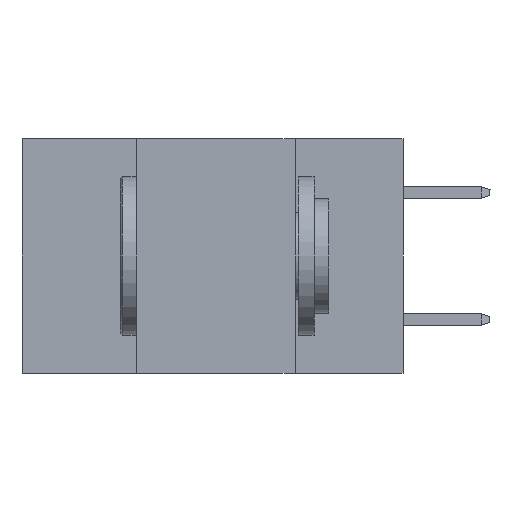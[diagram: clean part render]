
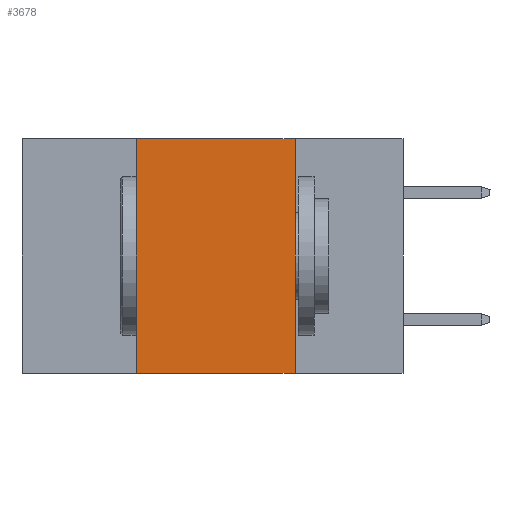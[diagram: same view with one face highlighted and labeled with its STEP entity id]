
A CAD part, left-side view. The second image highlights one B-rep face of the part: STEP entity #3678.
In plain terms, the highlighted planar face has unit normal (-1, 0, 0).
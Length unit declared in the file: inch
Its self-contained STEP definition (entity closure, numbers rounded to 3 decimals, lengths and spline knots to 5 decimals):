
#543 = ORIENTED_EDGE ( 'NONE', *, *, #1436, .F. ) ;
#1436 = EDGE_CURVE ( 'NONE', #8784, #13768, #17062, .T. ) ;
#1684 = DIRECTION ( 'NONE',  ( 1., 0., 0. ) ) ;
#2003 = CARTESIAN_POINT ( 'NONE',  ( 0., 0.42, 0. ) ) ;
#2241 = CARTESIAN_POINT ( 'NONE',  ( 0., 0.6, 0. ) ) ;
#2325 = EDGE_CURVE ( 'NONE', #8310, #11814, #17284, .T. ) ;
#3015 = PLANE ( 'NONE',  #15207 ) ;
#3678 = ADVANCED_FACE ( 'NONE', ( #11215 ), #3015, .F. ) ;
#4922 = LINE ( 'NONE', #2241, #7880 ) ;
#5837 = CARTESIAN_POINT ( 'NONE',  ( 0., 0.6, -0.37 ) ) ;
#6354 = VECTOR ( 'NONE', #16234, 39.37008 ) ;
#6727 = ORIENTED_EDGE ( 'NONE', *, *, #2325, .F. ) ;
#6838 = VECTOR ( 'NONE', #12905, 39.37008 ) ;
#7275 = ORIENTED_EDGE ( 'NONE', *, *, #7695, .T. ) ;
#7695 = EDGE_CURVE ( 'NONE', #8784, #11814, #16608, .T. ) ;
#7716 = DIRECTION ( 'NONE',  ( 0., -1., 0. ) ) ;
#7880 = VECTOR ( 'NONE', #7716, 39.37008 ) ;
#8310 = VERTEX_POINT ( 'NONE', #11149 ) ;
#8784 = VERTEX_POINT ( 'NONE', #8899 ) ;
#8899 = CARTESIAN_POINT ( 'NONE',  ( 0., 0.42, -0.37 ) ) ;
#9472 = CARTESIAN_POINT ( 'NONE',  ( 0., 0.17, 0. ) ) ;
#9924 = DIRECTION ( 'NONE',  ( 0., -1., 0. ) ) ;
#9996 = CARTESIAN_POINT ( 'NONE',  ( 0., 0.17, -0.37 ) ) ;
#10149 = CARTESIAN_POINT ( 'NONE',  ( 0., 0.6, 0. ) ) ;
#10281 = ORIENTED_EDGE ( 'NONE', *, *, #10549, .F. ) ;
#10549 = EDGE_CURVE ( 'NONE', #13768, #8310, #4922, .T. ) ;
#11149 = CARTESIAN_POINT ( 'NONE',  ( 0., 0.17, 0. ) ) ;
#11215 = FACE_OUTER_BOUND ( 'NONE', #13822, .T. ) ;
#11299 = DIRECTION ( 'NONE',  ( 0., 0., -1. ) ) ;
#11814 = VERTEX_POINT ( 'NONE', #9996 ) ;
#12905 = DIRECTION ( 'NONE',  ( 0., 0., 1. ) ) ;
#13768 = VERTEX_POINT ( 'NONE', #15091 ) ;
#13822 = EDGE_LOOP ( 'NONE', ( #6727, #10281, #543, #7275 ) ) ;
#15091 = CARTESIAN_POINT ( 'NONE',  ( 0., 0.42, 0. ) ) ;
#15207 = AXIS2_PLACEMENT_3D ( 'NONE', #10149, #1684, #11299 ) ;
#16149 = VECTOR ( 'NONE', #9924, 39.37008 ) ;
#16234 = DIRECTION ( 'NONE',  ( 0., 0., -1. ) ) ;
#16608 = LINE ( 'NONE', #5837, #16149 ) ;
#17062 = LINE ( 'NONE', #2003, #6838 ) ;
#17284 = LINE ( 'NONE', #9472, #6354 ) ;
